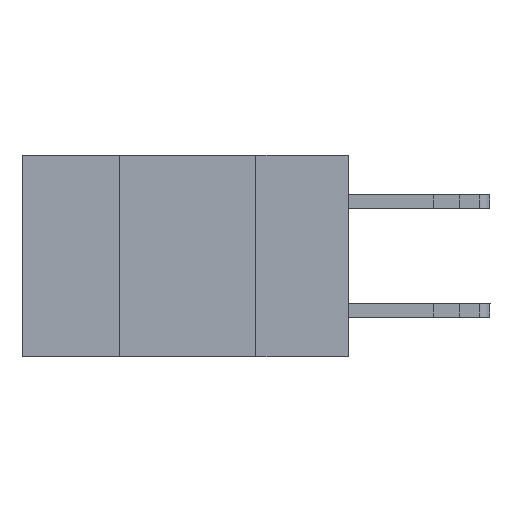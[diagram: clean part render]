
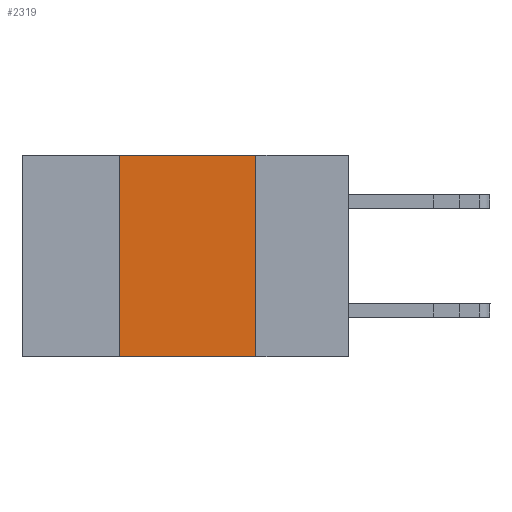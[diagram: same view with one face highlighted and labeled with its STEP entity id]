
A CAD part, left-side view. The second image highlights one B-rep face of the part: STEP entity #2319.
In plain terms, the highlighted planar face has unit normal (-1, 0, 0).
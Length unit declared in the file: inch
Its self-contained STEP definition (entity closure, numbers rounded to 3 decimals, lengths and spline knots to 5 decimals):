
#631 = EDGE_CURVE ( 'NONE', #11110, #10545, #10895, .T. ) ;
#1012 = ORIENTED_EDGE ( 'NONE', *, *, #3821, .F. ) ;
#1812 = VECTOR ( 'NONE', #9379, 39.37008 ) ;
#1994 = CARTESIAN_POINT ( 'NONE',  ( 0., 0.42, -0.37 ) ) ;
#2319 = ADVANCED_FACE ( 'NONE', ( #5328 ), #5441, .F. ) ;
#3821 = EDGE_CURVE ( 'NONE', #10545, #5839, #7639, .T. ) ;
#4053 = CARTESIAN_POINT ( 'NONE',  ( 0., 0.6, -0.37 ) ) ;
#4298 = DIRECTION ( 'NONE',  ( 0., -1., 0. ) ) ;
#4457 = CARTESIAN_POINT ( 'NONE',  ( 0., 0.6, 0. ) ) ;
#5328 = FACE_OUTER_BOUND ( 'NONE', #6663, .T. ) ;
#5423 = DIRECTION ( 'NONE',  ( 0., 0., -1. ) ) ;
#5427 = DIRECTION ( 'NONE',  ( 1., 0., 0. ) ) ;
#5441 = PLANE ( 'NONE',  #5673 ) ;
#5607 = CARTESIAN_POINT ( 'NONE',  ( 0., 0.6, 0. ) ) ;
#5673 = AXIS2_PLACEMENT_3D ( 'NONE', #5607, #5427, #5423 ) ;
#5839 = VERTEX_POINT ( 'NONE', #6144 ) ;
#6144 = CARTESIAN_POINT ( 'NONE',  ( 0., 0.17, 0. ) ) ;
#6497 = CARTESIAN_POINT ( 'NONE',  ( 0., 0.42, 0. ) ) ;
#6663 = EDGE_LOOP ( 'NONE', ( #8114, #1012, #10193, #9934 ) ) ;
#6712 = EDGE_CURVE ( 'NONE', #5839, #9380, #10053, .T. ) ;
#7505 = DIRECTION ( 'NONE',  ( 0., -1., 0. ) ) ;
#7639 = LINE ( 'NONE', #4457, #9728 ) ;
#7688 = VECTOR ( 'NONE', #11416, 39.37008 ) ;
#8114 = ORIENTED_EDGE ( 'NONE', *, *, #6712, .F. ) ;
#8929 = CARTESIAN_POINT ( 'NONE',  ( 0., 0.42, -0.37 ) ) ;
#9299 = LINE ( 'NONE', #4053, #11311 ) ;
#9379 = DIRECTION ( 'NONE',  ( 0., 0., 1. ) ) ;
#9380 = VERTEX_POINT ( 'NONE', #11415 ) ;
#9727 = CARTESIAN_POINT ( 'NONE',  ( 0., 0.17, -0.37 ) ) ;
#9728 = VECTOR ( 'NONE', #4298, 39.37008 ) ;
#9910 = EDGE_CURVE ( 'NONE', #11110, #9380, #9299, .T. ) ;
#9934 = ORIENTED_EDGE ( 'NONE', *, *, #9910, .T. ) ;
#10053 = LINE ( 'NONE', #9727, #7688 ) ;
#10193 = ORIENTED_EDGE ( 'NONE', *, *, #631, .F. ) ;
#10545 = VERTEX_POINT ( 'NONE', #6497 ) ;
#10895 = LINE ( 'NONE', #1994, #1812 ) ;
#11110 = VERTEX_POINT ( 'NONE', #8929 ) ;
#11311 = VECTOR ( 'NONE', #7505, 39.37008 ) ;
#11415 = CARTESIAN_POINT ( 'NONE',  ( 0., 0.17, -0.37 ) ) ;
#11416 = DIRECTION ( 'NONE',  ( 0., 0., -1. ) ) ;
